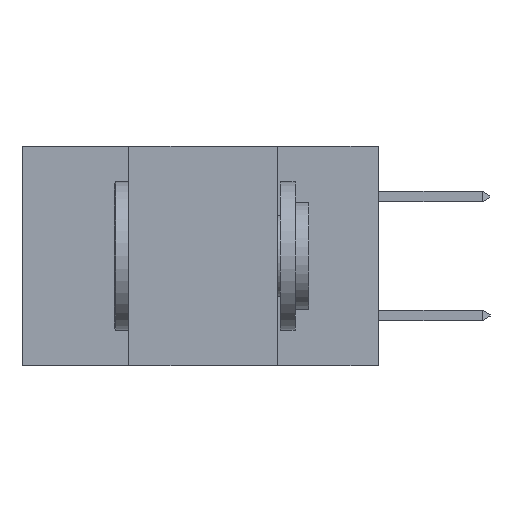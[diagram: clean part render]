
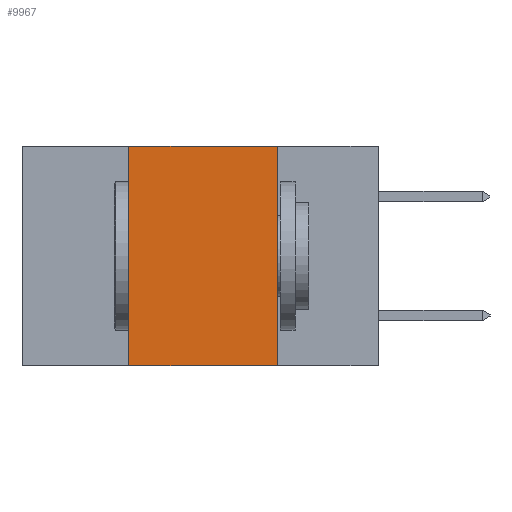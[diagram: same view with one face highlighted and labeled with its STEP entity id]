
A CAD part, left-side view. The second image highlights one B-rep face of the part: STEP entity #9967.
In plain terms, the highlighted planar face has unit normal (-1, 0, 0).
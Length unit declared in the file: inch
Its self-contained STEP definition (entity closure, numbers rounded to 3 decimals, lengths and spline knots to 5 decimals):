
#468 = EDGE_CURVE ( 'NONE', #13366, #9781, #3616, .T. ) ;
#562 = AXIS2_PLACEMENT_3D ( 'NONE', #2191, #1476, #4232 ) ;
#796 = VECTOR ( 'NONE', #5786, 39.37008 ) ;
#902 = ORIENTED_EDGE ( 'NONE', *, *, #4686, .T. ) ;
#1476 = DIRECTION ( 'NONE',  ( 1., 0., 0. ) ) ;
#1707 = VECTOR ( 'NONE', #11782, 39.37008 ) ;
#2149 = ORIENTED_EDGE ( 'NONE', *, *, #468, .F. ) ;
#2188 = PLANE ( 'NONE',  #562 ) ;
#2191 = CARTESIAN_POINT ( 'NONE',  ( 0., 0.6, 0. ) ) ;
#3563 = VECTOR ( 'NONE', #5867, 39.37008 ) ;
#3616 = LINE ( 'NONE', #4283, #9396 ) ;
#4232 = DIRECTION ( 'NONE',  ( 0., 0., -1. ) ) ;
#4283 = CARTESIAN_POINT ( 'NONE',  ( 0., 0.42, -0.37 ) ) ;
#4686 = EDGE_CURVE ( 'NONE', #13366, #14318, #6739, .T. ) ;
#4704 = CARTESIAN_POINT ( 'NONE',  ( 0., 0.17, 0. ) ) ;
#5020 = EDGE_LOOP ( 'NONE', ( #12912, #9384, #2149, #902 ) ) ;
#5383 = CARTESIAN_POINT ( 'NONE',  ( 0., 0.42, 0. ) ) ;
#5786 = DIRECTION ( 'NONE',  ( 0., 0., -1. ) ) ;
#5850 = CARTESIAN_POINT ( 'NONE',  ( 0., 0.17, -0.37 ) ) ;
#5867 = DIRECTION ( 'NONE',  ( 0., -1., 0. ) ) ;
#6295 = EDGE_CURVE ( 'NONE', #9781, #7437, #11181, .T. ) ;
#6739 = LINE ( 'NONE', #10529, #3563 ) ;
#7022 = LINE ( 'NONE', #5850, #796 ) ;
#7437 = VERTEX_POINT ( 'NONE', #4704 ) ;
#7705 = CARTESIAN_POINT ( 'NONE',  ( 0., 0.17, -0.37 ) ) ;
#9384 = ORIENTED_EDGE ( 'NONE', *, *, #6295, .F. ) ;
#9396 = VECTOR ( 'NONE', #9933, 39.37008 ) ;
#9781 = VERTEX_POINT ( 'NONE', #5383 ) ;
#9933 = DIRECTION ( 'NONE',  ( 0., 0., 1. ) ) ;
#9967 = ADVANCED_FACE ( 'NONE', ( #13382 ), #2188, .F. ) ;
#10529 = CARTESIAN_POINT ( 'NONE',  ( 0., 0.6, -0.37 ) ) ;
#11181 = LINE ( 'NONE', #14463, #1707 ) ;
#11782 = DIRECTION ( 'NONE',  ( 0., -1., 0. ) ) ;
#12912 = ORIENTED_EDGE ( 'NONE', *, *, #14570, .F. ) ;
#13366 = VERTEX_POINT ( 'NONE', #14490 ) ;
#13382 = FACE_OUTER_BOUND ( 'NONE', #5020, .T. ) ;
#14318 = VERTEX_POINT ( 'NONE', #7705 ) ;
#14463 = CARTESIAN_POINT ( 'NONE',  ( 0., 0.6, 0. ) ) ;
#14490 = CARTESIAN_POINT ( 'NONE',  ( 0., 0.42, -0.37 ) ) ;
#14570 = EDGE_CURVE ( 'NONE', #7437, #14318, #7022, .T. ) ;
